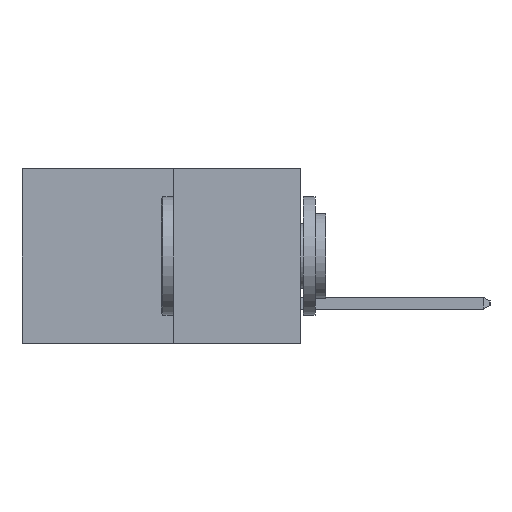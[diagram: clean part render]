
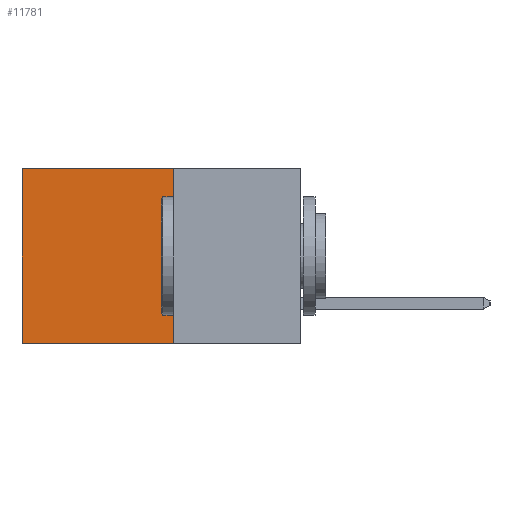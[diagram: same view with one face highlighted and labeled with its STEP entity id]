
A CAD part, left-side view. The second image highlights one B-rep face of the part: STEP entity #11781.
In plain terms, the highlighted planar face has unit normal (-1, 0, 0).
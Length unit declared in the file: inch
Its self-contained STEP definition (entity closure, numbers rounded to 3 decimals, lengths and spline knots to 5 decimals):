
#83 = LINE ( 'NONE', #6747, #11817 ) ;
#1024 = EDGE_CURVE ( 'NONE', #4716, #1522, #6207, .T. ) ;
#1041 = VECTOR ( 'NONE', #9043, 39.37008 ) ;
#1522 = VERTEX_POINT ( 'NONE', #9387 ) ;
#1855 = EDGE_LOOP ( 'NONE', ( #8863, #8779, #8803, #8940 ) ) ;
#2074 = DIRECTION ( 'NONE',  ( 0., 1., 0. ) ) ;
#3534 = VECTOR ( 'NONE', #2074, 39.37008 ) ;
#4250 = LINE ( 'NONE', #4544, #9934 ) ;
#4429 = EDGE_CURVE ( 'NONE', #8076, #7747, #8890, .T. ) ;
#4544 = CARTESIAN_POINT ( 'NONE',  ( 0.277, 0.27, -0.37 ) ) ;
#4594 = EDGE_CURVE ( 'NONE', #1522, #7747, #83, .T. ) ;
#4716 = VERTEX_POINT ( 'NONE', #5339 ) ;
#5097 = CARTESIAN_POINT ( 'NONE',  ( 0.277, 0.59, -0.37 ) ) ;
#5249 = DIRECTION ( 'NONE',  ( 0., 0., -1. ) ) ;
#5339 = CARTESIAN_POINT ( 'NONE',  ( 0.277, 0.27, 0. ) ) ;
#6207 = LINE ( 'NONE', #9883, #3534 ) ;
#6747 = CARTESIAN_POINT ( 'NONE',  ( 0.277, 0.59, -0.37 ) ) ;
#6957 = DIRECTION ( 'NONE',  ( 0., 0., -1. ) ) ;
#7747 = VERTEX_POINT ( 'NONE', #5097 ) ;
#8076 = VERTEX_POINT ( 'NONE', #10323 ) ;
#8779 = ORIENTED_EDGE ( 'NONE', *, *, #4429, .F. ) ;
#8803 = ORIENTED_EDGE ( 'NONE', *, *, #11955, .F. ) ;
#8863 = ORIENTED_EDGE ( 'NONE', *, *, #4594, .T. ) ;
#8890 = LINE ( 'NONE', #9109, #1041 ) ;
#8940 = ORIENTED_EDGE ( 'NONE', *, *, #1024, .T. ) ;
#9043 = DIRECTION ( 'NONE',  ( 0., 1., 0. ) ) ;
#9082 = CARTESIAN_POINT ( 'NONE',  ( 0.277, 0.27, -0.37 ) ) ;
#9109 = CARTESIAN_POINT ( 'NONE',  ( 0.277, 0.27, -0.37 ) ) ;
#9387 = CARTESIAN_POINT ( 'NONE',  ( 0.277, 0.59, 0. ) ) ;
#9883 = CARTESIAN_POINT ( 'NONE',  ( 0.277, 0.27, 0. ) ) ;
#9934 = VECTOR ( 'NONE', #11065, 39.37008 ) ;
#10323 = CARTESIAN_POINT ( 'NONE',  ( 0.277, 0.27, -0.37 ) ) ;
#10814 = DIRECTION ( 'NONE',  ( 1., 0., 0. ) ) ;
#11024 = AXIS2_PLACEMENT_3D ( 'NONE', #9082, #10814, #5249 ) ;
#11065 = DIRECTION ( 'NONE',  ( 0., 0., -1. ) ) ;
#11253 = FACE_OUTER_BOUND ( 'NONE', #1855, .T. ) ;
#11612 = PLANE ( 'NONE',  #11024 ) ;
#11781 = ADVANCED_FACE ( 'NONE', ( #11253 ), #11612, .F. ) ;
#11817 = VECTOR ( 'NONE', #6957, 39.37008 ) ;
#11955 = EDGE_CURVE ( 'NONE', #4716, #8076, #4250, .T. ) ;
